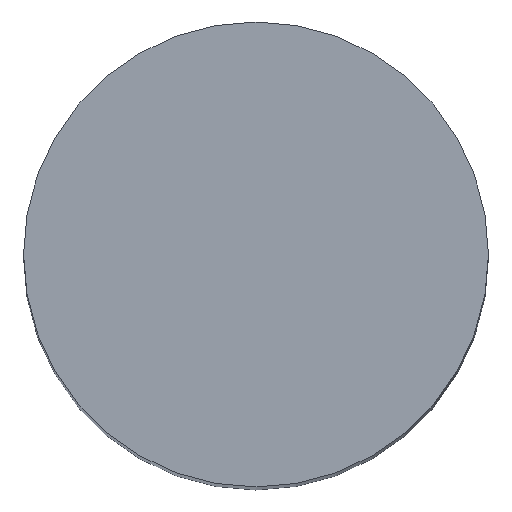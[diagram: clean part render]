
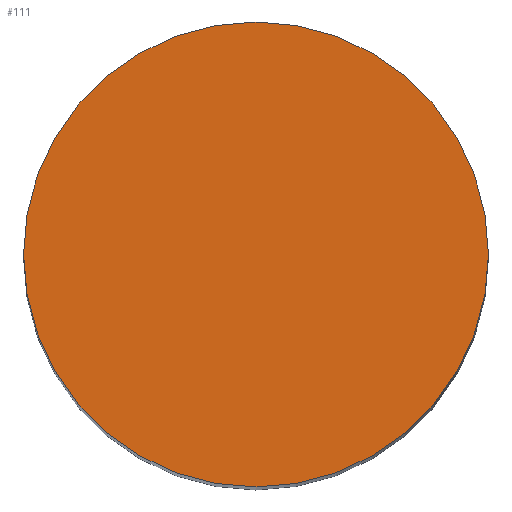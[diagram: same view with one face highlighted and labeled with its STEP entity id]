
A CAD part, top view. The second image highlights one B-rep face of the part: STEP entity #111.
In plain terms, the highlighted planar face has unit normal (0, 0, 1).
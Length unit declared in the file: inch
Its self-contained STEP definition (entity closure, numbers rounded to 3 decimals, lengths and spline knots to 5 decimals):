
#11 = EDGE_LOOP ( 'NONE', ( #118, #69 ) ) ;
#21 = DIRECTION ( 'NONE',  ( 0., 0., 1. ) ) ;
#22 = AXIS2_PLACEMENT_3D ( 'NONE', #110, #52, #120 ) ;
#27 = CARTESIAN_POINT ( 'NONE',  ( 0.11811, 0., 0.88583 ) ) ;
#38 = FACE_OUTER_BOUND ( 'NONE', #11, .T. ) ;
#48 = AXIS2_PLACEMENT_3D ( 'NONE', #108, #77, #53 ) ;
#50 = CIRCLE ( 'NONE', #58, 0.11811 ) ;
#52 = DIRECTION ( 'NONE',  ( 0., 0., 1. ) ) ;
#53 = DIRECTION ( 'NONE',  ( 1., 0., 0. ) ) ;
#58 = AXIS2_PLACEMENT_3D ( 'NONE', #94, #21, #101 ) ;
#69 = ORIENTED_EDGE ( 'NONE', *, *, #81, .T. ) ;
#75 = CARTESIAN_POINT ( 'NONE',  ( -0.11811, 0., 0.88583 ) ) ;
#77 = DIRECTION ( 'NONE',  ( 0., 0., 1. ) ) ;
#81 = EDGE_CURVE ( 'NONE', #83, #107, #85, .T. ) ;
#83 = VERTEX_POINT ( 'NONE', #27 ) ;
#85 = CIRCLE ( 'NONE', #48, 0.11811 ) ;
#86 = EDGE_CURVE ( 'NONE', #107, #83, #50, .T. ) ;
#94 = CARTESIAN_POINT ( 'NONE',  ( 0., 0., 0.88583 ) ) ;
#101 = DIRECTION ( 'NONE',  ( 1., 0., 0. ) ) ;
#107 = VERTEX_POINT ( 'NONE', #75 ) ;
#108 = CARTESIAN_POINT ( 'NONE',  ( 0., 0., 0.88583 ) ) ;
#110 = CARTESIAN_POINT ( 'NONE',  ( 0., 0., 0.88583 ) ) ;
#111 = ADVANCED_FACE ( 'NONE', ( #38 ), #147, .T. ) ;
#118 = ORIENTED_EDGE ( 'NONE', *, *, #86, .T. ) ;
#120 = DIRECTION ( 'NONE',  ( 1., 0., 0. ) ) ;
#147 = PLANE ( 'NONE',  #22 ) ;
